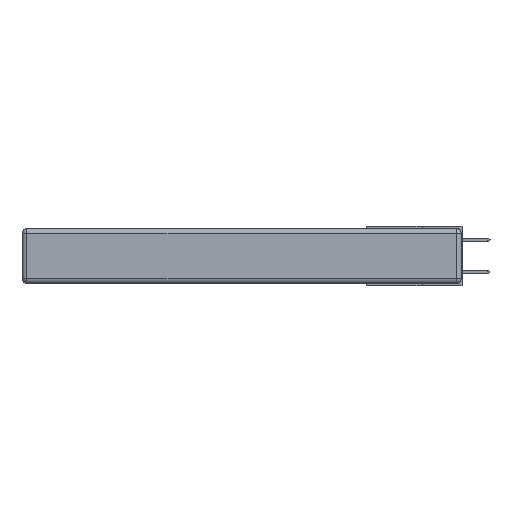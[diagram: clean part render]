
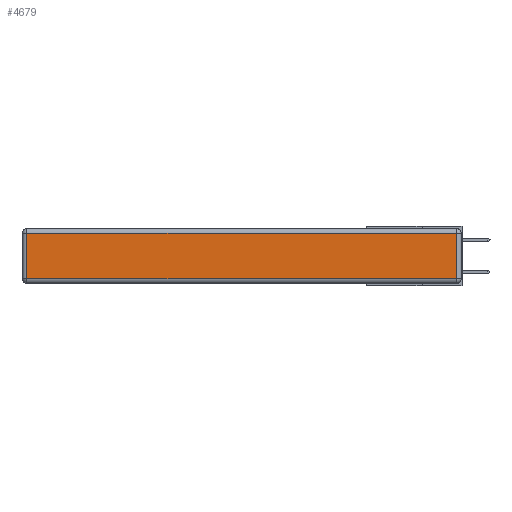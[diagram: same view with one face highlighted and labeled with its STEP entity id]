
A CAD part, left-side view. The second image highlights one B-rep face of the part: STEP entity #4679.
In plain terms, the highlighted planar face has unit normal (-1, 0, 0).
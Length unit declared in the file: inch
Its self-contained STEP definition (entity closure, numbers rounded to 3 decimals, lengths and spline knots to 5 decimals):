
#1350 = LINE ( 'NONE', #14559, #20274 ) ;
#1445 = EDGE_CURVE ( 'NONE', #11612, #3945, #1350, .T. ) ;
#1633 = DIRECTION ( 'NONE',  ( 0., 1., 0. ) ) ;
#1754 = EDGE_LOOP ( 'NONE', ( #16575, #22398, #15571, #14267 ) ) ;
#2818 = LINE ( 'NONE', #18284, #18293 ) ;
#3945 = VERTEX_POINT ( 'NONE', #12541 ) ;
#4679 = ADVANCED_FACE ( 'NONE', ( #19819 ), #16309, .T. ) ;
#5745 = CARTESIAN_POINT ( 'NONE',  ( 0., 0.03, -0.03 ) ) ;
#6007 = EDGE_CURVE ( 'NONE', #3945, #10282, #17616, .T. ) ;
#6945 = CARTESIAN_POINT ( 'NONE',  ( 0., 0., -0.313 ) ) ;
#7051 = DIRECTION ( 'NONE',  ( 0., 0., 1. ) ) ;
#7082 = CARTESIAN_POINT ( 'NONE',  ( 0., 0., -0.343 ) ) ;
#7239 = DIRECTION ( 'NONE',  ( 0., 0., 1. ) ) ;
#9328 = LINE ( 'NONE', #12602, #12755 ) ;
#10282 = VERTEX_POINT ( 'NONE', #10857 ) ;
#10303 = EDGE_CURVE ( 'NONE', #10282, #20621, #2818, .T. ) ;
#10857 = CARTESIAN_POINT ( 'NONE',  ( 0., 0.03, -0.313 ) ) ;
#11612 = VERTEX_POINT ( 'NONE', #15056 ) ;
#12541 = CARTESIAN_POINT ( 'NONE',  ( 0., 2.72, -0.313 ) ) ;
#12602 = CARTESIAN_POINT ( 'NONE',  ( 0., 2.75, -0.03 ) ) ;
#12755 = VECTOR ( 'NONE', #1633, 39.37008 ) ;
#13355 = AXIS2_PLACEMENT_3D ( 'NONE', #7082, #21786, #7239 ) ;
#14056 = DIRECTION ( 'NONE',  ( 0., -1., 0. ) ) ;
#14267 = ORIENTED_EDGE ( 'NONE', *, *, #1445, .T. ) ;
#14559 = CARTESIAN_POINT ( 'NONE',  ( 0., 2.72, -0.343 ) ) ;
#15056 = CARTESIAN_POINT ( 'NONE',  ( 0., 2.72, -0.03 ) ) ;
#15571 = ORIENTED_EDGE ( 'NONE', *, *, #16835, .T. ) ;
#16309 = PLANE ( 'NONE',  #13355 ) ;
#16575 = ORIENTED_EDGE ( 'NONE', *, *, #6007, .T. ) ;
#16835 = EDGE_CURVE ( 'NONE', #20621, #11612, #9328, .T. ) ;
#17616 = LINE ( 'NONE', #6945, #18782 ) ;
#18045 = DIRECTION ( 'NONE',  ( 0., 0., -1. ) ) ;
#18284 = CARTESIAN_POINT ( 'NONE',  ( 0., 0.03, -0.343 ) ) ;
#18293 = VECTOR ( 'NONE', #7051, 39.37008 ) ;
#18782 = VECTOR ( 'NONE', #14056, 39.37008 ) ;
#19819 = FACE_OUTER_BOUND ( 'NONE', #1754, .T. ) ;
#20274 = VECTOR ( 'NONE', #18045, 39.37008 ) ;
#20621 = VERTEX_POINT ( 'NONE', #5745 ) ;
#21786 = DIRECTION ( 'NONE',  ( -1., 0., 0. ) ) ;
#22398 = ORIENTED_EDGE ( 'NONE', *, *, #10303, .T. ) ;
